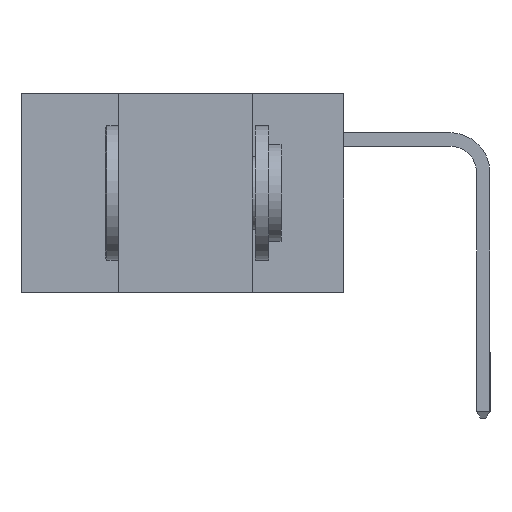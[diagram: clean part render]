
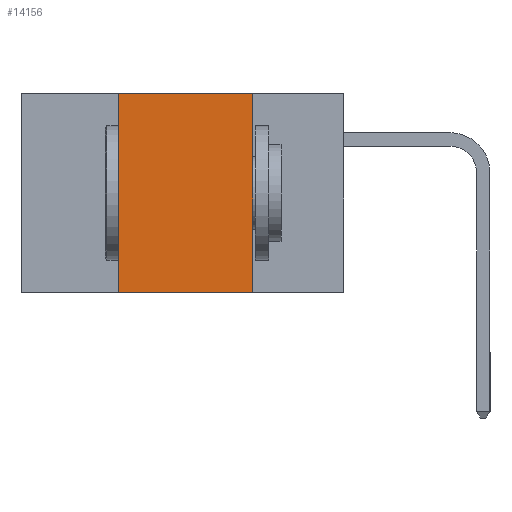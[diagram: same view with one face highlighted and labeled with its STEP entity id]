
A CAD part, left-side view. The second image highlights one B-rep face of the part: STEP entity #14156.
In plain terms, the highlighted planar face has unit normal (-1, 0, 0).
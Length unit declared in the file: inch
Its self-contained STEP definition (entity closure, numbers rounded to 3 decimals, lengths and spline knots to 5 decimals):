
#324 = DIRECTION ( 'NONE',  ( 0., 0., -1. ) ) ;
#491 = ORIENTED_EDGE ( 'NONE', *, *, #6171, .F. ) ;
#970 = DIRECTION ( 'NONE',  ( 0., 0., 1. ) ) ;
#2479 = DIRECTION ( 'NONE',  ( 0., 0., -1. ) ) ;
#2538 = VECTOR ( 'NONE', #324, 39.37008 ) ;
#4486 = DIRECTION ( 'NONE',  ( 0., -1., 0. ) ) ;
#5443 = DIRECTION ( 'NONE',  ( 1., 0., 0. ) ) ;
#6171 = EDGE_CURVE ( 'NONE', #9457, #16876, #8784, .T. ) ;
#7531 = DIRECTION ( 'NONE',  ( 0., -1., 0. ) ) ;
#7594 = CARTESIAN_POINT ( 'NONE',  ( 0., 0.6, 0. ) ) ;
#8176 = EDGE_CURVE ( 'NONE', #14639, #14981, #16053, .T. ) ;
#8338 = CARTESIAN_POINT ( 'NONE',  ( 0., 0.42, 0. ) ) ;
#8679 = CARTESIAN_POINT ( 'NONE',  ( 0., 0.17, -0.37 ) ) ;
#8784 = LINE ( 'NONE', #15170, #2538 ) ;
#9291 = ORIENTED_EDGE ( 'NONE', *, *, #11836, .T. ) ;
#9457 = VERTEX_POINT ( 'NONE', #12391 ) ;
#10127 = LINE ( 'NONE', #7594, #14549 ) ;
#10837 = CARTESIAN_POINT ( 'NONE',  ( 0., 0.42, -0.37 ) ) ;
#11196 = CARTESIAN_POINT ( 'NONE',  ( 0., 0.6, 0. ) ) ;
#11384 = ORIENTED_EDGE ( 'NONE', *, *, #8176, .F. ) ;
#11836 = EDGE_CURVE ( 'NONE', #14639, #16876, #15935, .T. ) ;
#12391 = CARTESIAN_POINT ( 'NONE',  ( 0., 0.17, 0. ) ) ;
#13320 = AXIS2_PLACEMENT_3D ( 'NONE', #11196, #5443, #2479 ) ;
#13497 = EDGE_CURVE ( 'NONE', #14981, #9457, #10127, .T. ) ;
#13832 = EDGE_LOOP ( 'NONE', ( #491, #16033, #11384, #9291 ) ) ;
#14060 = VECTOR ( 'NONE', #4486, 39.37008 ) ;
#14156 = ADVANCED_FACE ( 'NONE', ( #14530 ), #14199, .F. ) ;
#14199 = PLANE ( 'NONE',  #13320 ) ;
#14530 = FACE_OUTER_BOUND ( 'NONE', #13832, .T. ) ;
#14549 = VECTOR ( 'NONE', #7531, 39.37008 ) ;
#14639 = VERTEX_POINT ( 'NONE', #10837 ) ;
#14981 = VERTEX_POINT ( 'NONE', #17844 ) ;
#15170 = CARTESIAN_POINT ( 'NONE',  ( 0., 0.17, 0. ) ) ;
#15935 = LINE ( 'NONE', #19205, #14060 ) ;
#16033 = ORIENTED_EDGE ( 'NONE', *, *, #13497, .F. ) ;
#16053 = LINE ( 'NONE', #8338, #17626 ) ;
#16876 = VERTEX_POINT ( 'NONE', #8679 ) ;
#17626 = VECTOR ( 'NONE', #970, 39.37008 ) ;
#17844 = CARTESIAN_POINT ( 'NONE',  ( 0., 0.42, 0. ) ) ;
#19205 = CARTESIAN_POINT ( 'NONE',  ( 0., 0.6, -0.37 ) ) ;
